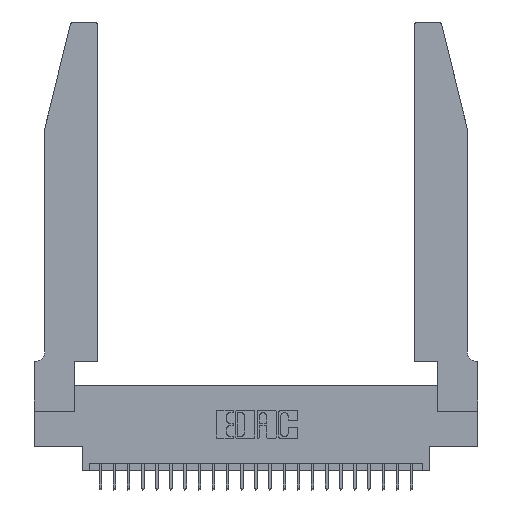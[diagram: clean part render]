
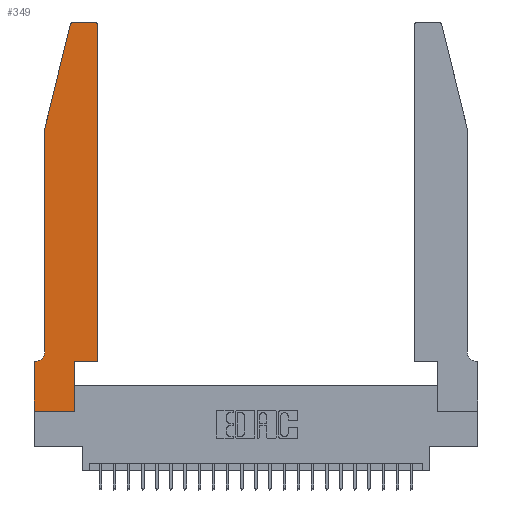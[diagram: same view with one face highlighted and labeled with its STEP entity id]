
A CAD part, top view. The second image highlights one B-rep face of the part: STEP entity #349.
In plain terms, the highlighted planar face has unit normal (0, 0, 1).
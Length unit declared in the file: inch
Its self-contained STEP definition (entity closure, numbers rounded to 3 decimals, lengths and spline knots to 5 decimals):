
#43 = DIRECTION ( 'NONE',  ( -1., 0., 0. ) ) ;
#131 = EDGE_CURVE ( 'NONE', #6403, #14922, #13853, .T. ) ;
#149 = DIRECTION ( 'NONE',  ( 1., 0., 0. ) ) ;
#159 = CARTESIAN_POINT ( 'NONE',  ( 0.4505, 0.35, 0.37 ) ) ;
#245 = ORIENTED_EDGE ( 'NONE', *, *, #131, .T. ) ;
#271 = ORIENTED_EDGE ( 'NONE', *, *, #23717, .T. ) ;
#349 = ADVANCED_FACE ( 'NONE', ( #21243 ), #3474, .T. ) ;
#386 = CARTESIAN_POINT ( 'NONE',  ( 0.4205, 2.75, 0.37 ) ) ;
#489 = CARTESIAN_POINT ( 'NONE',  ( 0.2865, 0.35, 0.37 ) ) ;
#1149 = LINE ( 'NONE', #7023, #17305 ) ;
#1385 = DIRECTION ( 'NONE',  ( 0., 0., 1. ) ) ;
#1946 = ORIENTED_EDGE ( 'NONE', *, *, #5329, .T. ) ;
#2067 = VERTEX_POINT ( 'NONE', #25109 ) ;
#2417 = CARTESIAN_POINT ( 'NONE',  ( 0.4505, 0.35, 0.37 ) ) ;
#2438 = VECTOR ( 'NONE', #24248, 39.37008 ) ;
#2697 = VECTOR ( 'NONE', #5821, 39.37008 ) ;
#2731 = LINE ( 'NONE', #16344, #2438 ) ;
#3474 = PLANE ( 'NONE',  #11704 ) ;
#3626 = CARTESIAN_POINT ( 'NONE',  ( 0.0755, 2., 0.37 ) ) ;
#3656 = VERTEX_POINT ( 'NONE', #2417 ) ;
#4008 = CARTESIAN_POINT ( 'NONE',  ( 0.2865, 0.35, 0.37 ) ) ;
#4472 = CARTESIAN_POINT ( 'NONE',  ( 0.4205, 2.72, 0.37 ) ) ;
#4638 = ORIENTED_EDGE ( 'NONE', *, *, #7424, .T. ) ;
#4687 = DIRECTION ( 'NONE',  ( -1., 0., 0. ) ) ;
#4996 = EDGE_CURVE ( 'NONE', #14922, #3656, #6237, .T. ) ;
#5035 = VECTOR ( 'NONE', #23527, 39.37008 ) ;
#5118 = VERTEX_POINT ( 'NONE', #386 ) ;
#5306 = EDGE_LOOP ( 'NONE', ( #16510, #16017, #10654, #1946, #271, #6981, #24573, #4638, #245, #12256, #11789, #11338 ) ) ;
#5329 = EDGE_CURVE ( 'NONE', #6782, #20176, #17723, .T. ) ;
#5821 = DIRECTION ( 'NONE',  ( 0., -1., 0. ) ) ;
#6141 = DIRECTION ( 'NONE',  ( 0., 0., 1. ) ) ;
#6237 = LINE ( 'NONE', #7680, #13448 ) ;
#6403 = VERTEX_POINT ( 'NONE', #17231 ) ;
#6443 = LINE ( 'NONE', #9016, #14872 ) ;
#6782 = VERTEX_POINT ( 'NONE', #13058 ) ;
#6850 = VERTEX_POINT ( 'NONE', #19156 ) ;
#6981 = ORIENTED_EDGE ( 'NONE', *, *, #13584, .T. ) ;
#7023 = CARTESIAN_POINT ( 'NONE',  ( 0.0755, 0.35, 0.37 ) ) ;
#7389 = VERTEX_POINT ( 'NONE', #13295 ) ;
#7424 = EDGE_CURVE ( 'NONE', #6850, #6403, #19645, .T. ) ;
#7680 = CARTESIAN_POINT ( 'NONE',  ( 0.4505, 0.35, 0.37 ) ) ;
#7732 = CIRCLE ( 'NONE', #13509, 0.03 ) ;
#8173 = EDGE_CURVE ( 'NONE', #5118, #11263, #24368, .T. ) ;
#8188 = DIRECTION ( 'NONE',  ( 0., 1., 0. ) ) ;
#8437 = CARTESIAN_POINT ( 'NONE',  ( 0.25487, 2.72718, 0.37 ) ) ;
#8630 = DIRECTION ( 'NONE',  ( -0.239, -0.971, 0. ) ) ;
#9016 = CARTESIAN_POINT ( 'NONE',  ( 0.0755, 2., 0.37 ) ) ;
#9077 = DIRECTION ( 'NONE',  ( -1., 0., 0. ) ) ;
#9539 = CARTESIAN_POINT ( 'NONE',  ( 0., 0., 0.37 ) ) ;
#9630 = VECTOR ( 'NONE', #25384, 39.37008 ) ;
#9872 = CIRCLE ( 'NONE', #21641, 0.03 ) ;
#9933 = EDGE_CURVE ( 'NONE', #11263, #19628, #7732, .T. ) ;
#10265 = DIRECTION ( 'NONE',  ( 0., 0., -1. ) ) ;
#10654 = ORIENTED_EDGE ( 'NONE', *, *, #15521, .T. ) ;
#11263 = VERTEX_POINT ( 'NONE', #23293 ) ;
#11338 = ORIENTED_EDGE ( 'NONE', *, *, #23256, .T. ) ;
#11704 = AXIS2_PLACEMENT_3D ( 'NONE', #20855, #1385, #18885 ) ;
#11789 = ORIENTED_EDGE ( 'NONE', *, *, #14419, .T. ) ;
#12256 = ORIENTED_EDGE ( 'NONE', *, *, #4996, .T. ) ;
#12779 = CIRCLE ( 'NONE', #21082, 0.07 ) ;
#13058 = CARTESIAN_POINT ( 'NONE',  ( 0.0755, 2., 0.37 ) ) ;
#13295 = CARTESIAN_POINT ( 'NONE',  ( 0.0055, 0.35, 0.37 ) ) ;
#13448 = VECTOR ( 'NONE', #149, 39.37008 ) ;
#13509 = AXIS2_PLACEMENT_3D ( 'NONE', #14157, #6141, #24014 ) ;
#13584 = EDGE_CURVE ( 'NONE', #7389, #23195, #1149, .T. ) ;
#13740 = VECTOR ( 'NONE', #4687, 39.37008 ) ;
#13853 = LINE ( 'NONE', #4008, #9630 ) ;
#14059 = DIRECTION ( 'NONE',  ( 0., 0., 1. ) ) ;
#14157 = CARTESIAN_POINT ( 'NONE',  ( 0.284, 2.72, 0.37 ) ) ;
#14419 = EDGE_CURVE ( 'NONE', #3656, #2067, #15951, .T. ) ;
#14528 = CARTESIAN_POINT ( 'NONE',  ( 0.2605, 2.75, 0.37 ) ) ;
#14872 = VECTOR ( 'NONE', #8630, 39.37008 ) ;
#14922 = VERTEX_POINT ( 'NONE', #489 ) ;
#15249 = VECTOR ( 'NONE', #8188, 39.37008 ) ;
#15521 = EDGE_CURVE ( 'NONE', #19628, #6782, #6443, .T. ) ;
#15951 = LINE ( 'NONE', #159, #15249 ) ;
#16017 = ORIENTED_EDGE ( 'NONE', *, *, #9933, .T. ) ;
#16093 = CARTESIAN_POINT ( 'NONE',  ( 0.0055, 0.42, 0.37 ) ) ;
#16344 = CARTESIAN_POINT ( 'NONE',  ( 0., 0., 0.37 ) ) ;
#16510 = ORIENTED_EDGE ( 'NONE', *, *, #8173, .T. ) ;
#17231 = CARTESIAN_POINT ( 'NONE',  ( 0.2865, 0., 0.37 ) ) ;
#17305 = VECTOR ( 'NONE', #9077, 39.37008 ) ;
#17723 = LINE ( 'NONE', #3626, #2697 ) ;
#18885 = DIRECTION ( 'NONE',  ( 1., 0., 0. ) ) ;
#19156 = CARTESIAN_POINT ( 'NONE',  ( 0., 0., 0.37 ) ) ;
#19628 = VERTEX_POINT ( 'NONE', #8437 ) ;
#19645 = LINE ( 'NONE', #9539, #5035 ) ;
#20176 = VERTEX_POINT ( 'NONE', #21102 ) ;
#20855 = CARTESIAN_POINT ( 'NONE',  ( 0., 0.35, 0.37 ) ) ;
#21082 = AXIS2_PLACEMENT_3D ( 'NONE', #16093, #10265, #43 ) ;
#21102 = CARTESIAN_POINT ( 'NONE',  ( 0.0755, 0.42, 0.37 ) ) ;
#21243 = FACE_OUTER_BOUND ( 'NONE', #5306, .T. ) ;
#21641 = AXIS2_PLACEMENT_3D ( 'NONE', #4472, #14059, #21985 ) ;
#21985 = DIRECTION ( 'NONE',  ( 1., 0., 0. ) ) ;
#23195 = VERTEX_POINT ( 'NONE', #25590 ) ;
#23256 = EDGE_CURVE ( 'NONE', #2067, #5118, #9872, .T. ) ;
#23293 = CARTESIAN_POINT ( 'NONE',  ( 0.284, 2.75, 0.37 ) ) ;
#23527 = DIRECTION ( 'NONE',  ( 1., 0., 0. ) ) ;
#23717 = EDGE_CURVE ( 'NONE', #20176, #7389, #12779, .T. ) ;
#23883 = EDGE_CURVE ( 'NONE', #23195, #6850, #2731, .T. ) ;
#24014 = DIRECTION ( 'NONE',  ( 1., 0., 0. ) ) ;
#24248 = DIRECTION ( 'NONE',  ( 0., -1., 0. ) ) ;
#24368 = LINE ( 'NONE', #14528, #13740 ) ;
#24573 = ORIENTED_EDGE ( 'NONE', *, *, #23883, .T. ) ;
#25109 = CARTESIAN_POINT ( 'NONE',  ( 0.4505, 2.72, 0.37 ) ) ;
#25384 = DIRECTION ( 'NONE',  ( 0., 1., 0. ) ) ;
#25590 = CARTESIAN_POINT ( 'NONE',  ( 0., 0.35, 0.37 ) ) ;
